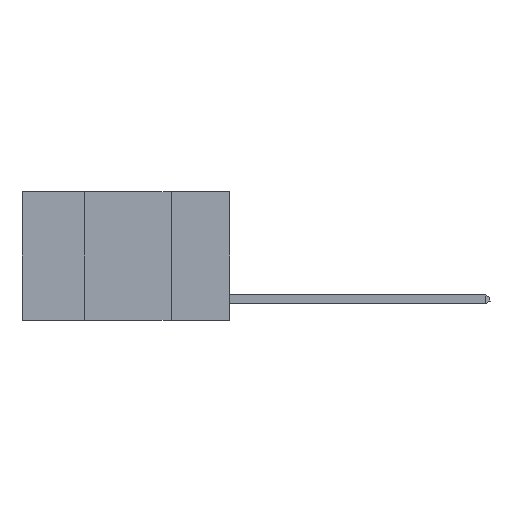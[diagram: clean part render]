
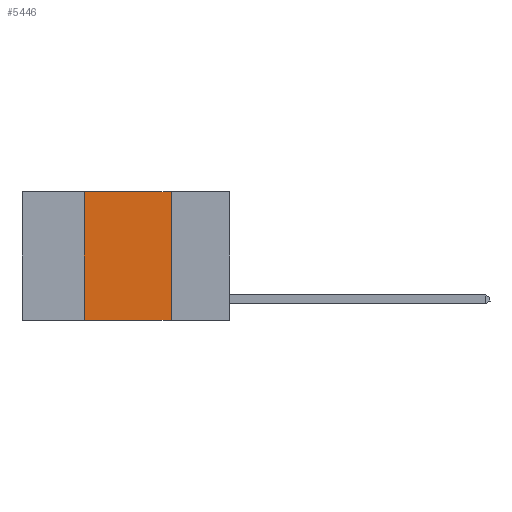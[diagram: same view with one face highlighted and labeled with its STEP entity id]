
A CAD part, left-side view. The second image highlights one B-rep face of the part: STEP entity #5446.
In plain terms, the highlighted planar face has unit normal (-1, 0, 0).
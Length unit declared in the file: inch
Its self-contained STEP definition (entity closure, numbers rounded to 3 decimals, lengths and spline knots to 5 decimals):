
#276 = EDGE_CURVE ( 'NONE', #5785, #2599, #2001, .T. ) ;
#340 = VERTEX_POINT ( 'NONE', #8635 ) ;
#548 = DIRECTION ( 'NONE',  ( 0., -1., 0. ) ) ;
#1341 = ORIENTED_EDGE ( 'NONE', *, *, #7193, .T. ) ;
#1648 = EDGE_CURVE ( 'NONE', #340, #9764, #4008, .T. ) ;
#1796 = LINE ( 'NONE', #3510, #6704 ) ;
#2001 = LINE ( 'NONE', #8324, #6705 ) ;
#2182 = EDGE_CURVE ( 'NONE', #9764, #5785, #1796, .T. ) ;
#2599 = VERTEX_POINT ( 'NONE', #8968 ) ;
#3204 = ORIENTED_EDGE ( 'NONE', *, *, #1648, .F. ) ;
#3510 = CARTESIAN_POINT ( 'NONE',  ( 0., 0.6, 0. ) ) ;
#3522 = CARTESIAN_POINT ( 'NONE',  ( 0., 0.17, 0. ) ) ;
#3751 = VECTOR ( 'NONE', #548, 39.37008 ) ;
#3763 = ORIENTED_EDGE ( 'NONE', *, *, #276, .F. ) ;
#3950 = DIRECTION ( 'NONE',  ( 0., 0., 1. ) ) ;
#4008 = LINE ( 'NONE', #8685, #5864 ) ;
#4219 = CARTESIAN_POINT ( 'NONE',  ( 0., 0.42, 0. ) ) ;
#4581 = CARTESIAN_POINT ( 'NONE',  ( 0., 0.6, 0. ) ) ;
#4729 = DIRECTION ( 'NONE',  ( 0., 0., -1. ) ) ;
#4924 = DIRECTION ( 'NONE',  ( 0., -1., 0. ) ) ;
#5446 = ADVANCED_FACE ( 'NONE', ( #7848 ), #9453, .F. ) ;
#5785 = VERTEX_POINT ( 'NONE', #3522 ) ;
#5802 = EDGE_LOOP ( 'NONE', ( #3763, #8034, #3204, #1341 ) ) ;
#5864 = VECTOR ( 'NONE', #3950, 39.37008 ) ;
#6561 = AXIS2_PLACEMENT_3D ( 'NONE', #4581, #9354, #4729 ) ;
#6704 = VECTOR ( 'NONE', #4924, 39.37008 ) ;
#6705 = VECTOR ( 'NONE', #8946, 39.37008 ) ;
#7193 = EDGE_CURVE ( 'NONE', #340, #2599, #7546, .T. ) ;
#7546 = LINE ( 'NONE', #9868, #3751 ) ;
#7848 = FACE_OUTER_BOUND ( 'NONE', #5802, .T. ) ;
#8034 = ORIENTED_EDGE ( 'NONE', *, *, #2182, .F. ) ;
#8324 = CARTESIAN_POINT ( 'NONE',  ( 0., 0.17, 0. ) ) ;
#8635 = CARTESIAN_POINT ( 'NONE',  ( 0., 0.42, -0.37 ) ) ;
#8685 = CARTESIAN_POINT ( 'NONE',  ( 0., 0.42, 0. ) ) ;
#8946 = DIRECTION ( 'NONE',  ( 0., 0., -1. ) ) ;
#8968 = CARTESIAN_POINT ( 'NONE',  ( 0., 0.17, -0.37 ) ) ;
#9354 = DIRECTION ( 'NONE',  ( 1., 0., 0. ) ) ;
#9453 = PLANE ( 'NONE',  #6561 ) ;
#9764 = VERTEX_POINT ( 'NONE', #4219 ) ;
#9868 = CARTESIAN_POINT ( 'NONE',  ( 0., 0.6, -0.37 ) ) ;
